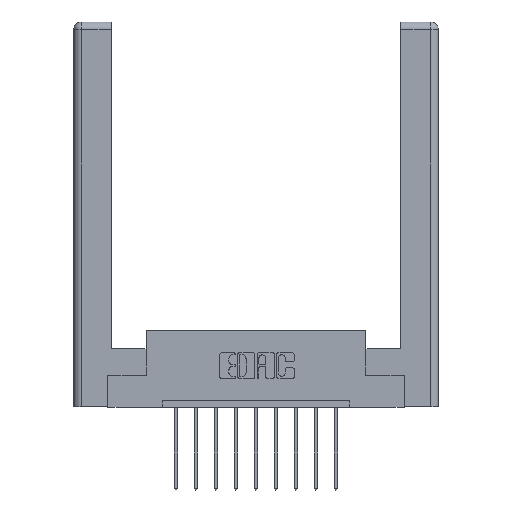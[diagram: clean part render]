
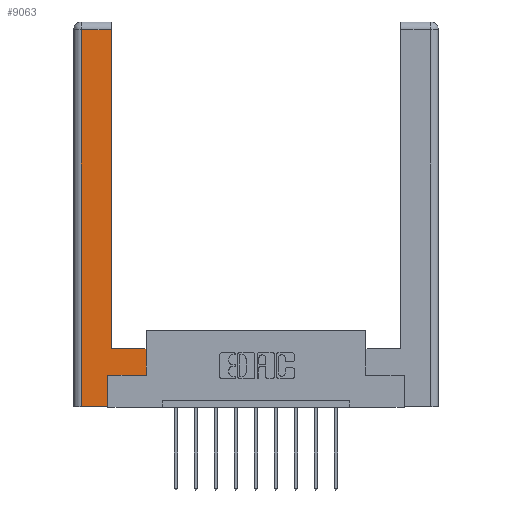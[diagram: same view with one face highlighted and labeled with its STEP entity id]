
A CAD part, top view. The second image highlights one B-rep face of the part: STEP entity #9063.
In plain terms, the highlighted planar face has unit normal (0, 0, 1).
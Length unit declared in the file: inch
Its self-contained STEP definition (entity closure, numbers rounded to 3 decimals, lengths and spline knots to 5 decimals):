
#66 = LINE ( 'NONE', #13144, #13555 ) ;
#110 = VERTEX_POINT ( 'NONE', #11685 ) ;
#160 = CARTESIAN_POINT ( 'NONE',  ( 0.265, 0., 0. ) ) ;
#459 = CARTESIAN_POINT ( 'NONE',  ( 0.265, 0.245, 0. ) ) ;
#613 = EDGE_CURVE ( 'NONE', #12065, #110, #4809, .T. ) ;
#688 = VERTEX_POINT ( 'NONE', #6399 ) ;
#804 = CARTESIAN_POINT ( 'NONE',  ( 0.0615, 0., 0. ) ) ;
#1315 = LINE ( 'NONE', #459, #6425 ) ;
#1377 = DIRECTION ( 'NONE',  ( 0., 1., 0. ) ) ;
#1468 = LINE ( 'NONE', #6371, #4754 ) ;
#1792 = CARTESIAN_POINT ( 'NONE',  ( 0.565, 0.45, 0. ) ) ;
#1894 = DIRECTION ( 'NONE',  ( 0., -1., 0. ) ) ;
#2212 = FACE_OUTER_BOUND ( 'NONE', #7364, .T. ) ;
#2738 = VERTEX_POINT ( 'NONE', #1792 ) ;
#2864 = DIRECTION ( 'NONE',  ( 0., 1., 0. ) ) ;
#2990 = ORIENTED_EDGE ( 'NONE', *, *, #4036, .T. ) ;
#3117 = ORIENTED_EDGE ( 'NONE', *, *, #7483, .T. ) ;
#3142 = CARTESIAN_POINT ( 'NONE',  ( 0.295, 3., 0. ) ) ;
#3475 = LINE ( 'NONE', #160, #12037 ) ;
#3572 = EDGE_CURVE ( 'NONE', #5681, #688, #1468, .T. ) ;
#3655 = EDGE_CURVE ( 'NONE', #10911, #5681, #1315, .T. ) ;
#4036 = EDGE_CURVE ( 'NONE', #110, #10911, #3475, .T. ) ;
#4037 = PLANE ( 'NONE',  #7356 ) ;
#4188 = VECTOR ( 'NONE', #7342, 39.37008 ) ;
#4458 = DIRECTION ( 'NONE',  ( -1., 0., 0. ) ) ;
#4754 = VECTOR ( 'NONE', #9872, 39.37008 ) ;
#4809 = LINE ( 'NONE', #804, #11759 ) ;
#5291 = DIRECTION ( 'NONE',  ( -1., 0., 0. ) ) ;
#5361 = ORIENTED_EDGE ( 'NONE', *, *, #3655, .T. ) ;
#5579 = ORIENTED_EDGE ( 'NONE', *, *, #8567, .T. ) ;
#5681 = VERTEX_POINT ( 'NONE', #12258 ) ;
#5795 = ORIENTED_EDGE ( 'NONE', *, *, #613, .T. ) ;
#6371 = CARTESIAN_POINT ( 'NONE',  ( 0.565, 0.245, 0. ) ) ;
#6399 = CARTESIAN_POINT ( 'NONE',  ( 0.565, 0.245, 0. ) ) ;
#6425 = VECTOR ( 'NONE', #1377, 39.37008 ) ;
#6557 = EDGE_CURVE ( 'NONE', #8006, #12065, #10479, .T. ) ;
#7332 = VECTOR ( 'NONE', #5291, 39.37008 ) ;
#7342 = DIRECTION ( 'NONE',  ( 0., 1., 0. ) ) ;
#7356 = AXIS2_PLACEMENT_3D ( 'NONE', #13462, #10403, #13414 ) ;
#7364 = EDGE_LOOP ( 'NONE', ( #8122, #9520, #5795, #2990, #5361, #13291, #5579, #3117 ) ) ;
#7483 = EDGE_CURVE ( 'NONE', #2738, #13199, #10448, .T. ) ;
#7596 = DIRECTION ( 'NONE',  ( 1., 0., 0. ) ) ;
#7599 = CARTESIAN_POINT ( 'NONE',  ( 0.0615, 2.94, 0. ) ) ;
#8006 = VERTEX_POINT ( 'NONE', #12493 ) ;
#8122 = ORIENTED_EDGE ( 'NONE', *, *, #8197, .T. ) ;
#8192 = VECTOR ( 'NONE', #4458, 39.37008 ) ;
#8197 = EDGE_CURVE ( 'NONE', #13199, #8006, #9631, .T. ) ;
#8567 = EDGE_CURVE ( 'NONE', #688, #2738, #66, .T. ) ;
#8752 = CARTESIAN_POINT ( 'NONE',  ( 0.0615, 2.94, 0. ) ) ;
#9011 = CARTESIAN_POINT ( 'NONE',  ( 0.265, 0., 0. ) ) ;
#9063 = ADVANCED_FACE ( 'NONE', ( #2212 ), #4037, .F. ) ;
#9520 = ORIENTED_EDGE ( 'NONE', *, *, #6557, .T. ) ;
#9631 = LINE ( 'NONE', #3142, #4188 ) ;
#9872 = DIRECTION ( 'NONE',  ( 1., 0., 0. ) ) ;
#10403 = DIRECTION ( 'NONE',  ( 0., 0., -1. ) ) ;
#10448 = LINE ( 'NONE', #11602, #7332 ) ;
#10479 = LINE ( 'NONE', #8752, #8192 ) ;
#10911 = VERTEX_POINT ( 'NONE', #9011 ) ;
#11602 = CARTESIAN_POINT ( 'NONE',  ( 0.295, 0.45, 0. ) ) ;
#11685 = CARTESIAN_POINT ( 'NONE',  ( 0.0615, 0., 0. ) ) ;
#11759 = VECTOR ( 'NONE', #1894, 39.37008 ) ;
#12037 = VECTOR ( 'NONE', #7596, 39.37008 ) ;
#12065 = VERTEX_POINT ( 'NONE', #7599 ) ;
#12258 = CARTESIAN_POINT ( 'NONE',  ( 0.265, 0.245, 0. ) ) ;
#12493 = CARTESIAN_POINT ( 'NONE',  ( 0.295, 2.94, 0. ) ) ;
#12781 = CARTESIAN_POINT ( 'NONE',  ( 0.295, 0.45, 0. ) ) ;
#13144 = CARTESIAN_POINT ( 'NONE',  ( 0.565, 0.45, 0. ) ) ;
#13199 = VERTEX_POINT ( 'NONE', #12781 ) ;
#13291 = ORIENTED_EDGE ( 'NONE', *, *, #3572, .T. ) ;
#13414 = DIRECTION ( 'NONE',  ( -1., 0., 0. ) ) ;
#13462 = CARTESIAN_POINT ( 'NONE',  ( 0., 0., 0. ) ) ;
#13555 = VECTOR ( 'NONE', #2864, 39.37008 ) ;
